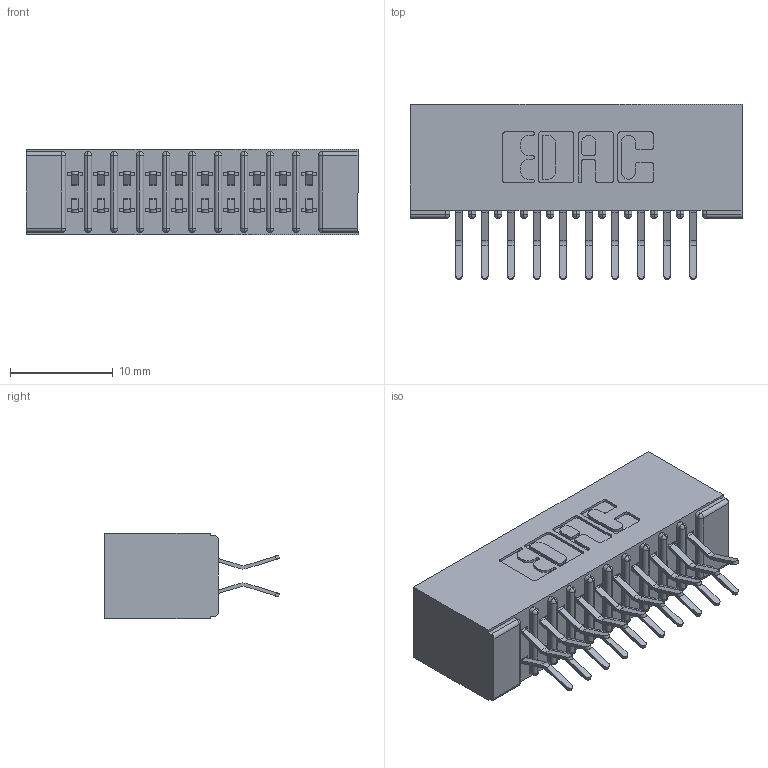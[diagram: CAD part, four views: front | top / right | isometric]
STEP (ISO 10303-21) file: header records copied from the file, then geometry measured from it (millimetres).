
FILE_DESCRIPTION (( 'STEP AP203' ), '1' );
FILE_NAME ('391-020-556-201.STEP', '2018-08-08T18:58:58', ( '' ), ( '' ), 'SwSTEP 2.0', 'SolidWorks 2016', '' );
FILE_SCHEMA (( 'CONFIG_CONTROL_DESIGN' ));
Length unit declared in the file: inch
Products named in the file (3): 341 Part_No Mounting Lugs; 341-292-001_341-292-156; 391-020-556-201
Assembly tree (21 placements, depth 2):
  391-020-556-201
    341 Part_No Mounting Lugs
    341-292-001_341-292-156  x20
Bounding box: 32.38 x 17.07 x 8.38 mm (x, y, z)
Volume: 2011.6 mm3; surface area: 4173 mm2
Topology: 21 solids, 21 shells, 1508 faces, 4362 edges, 2830 vertices
Faces by surface type: plane 864, cylinder 604, sphere 22, torus 18
Entity records: 16227 total; most frequent: CARTESIAN_POINT 2698, ORIENTED_EDGE 2676, DIRECTION 2644, EDGE_CURVE 1338, LINE 1044, VECTOR 1044, VERTEX_POINT 854, AXIS2_PLACEMENT_3D 800
